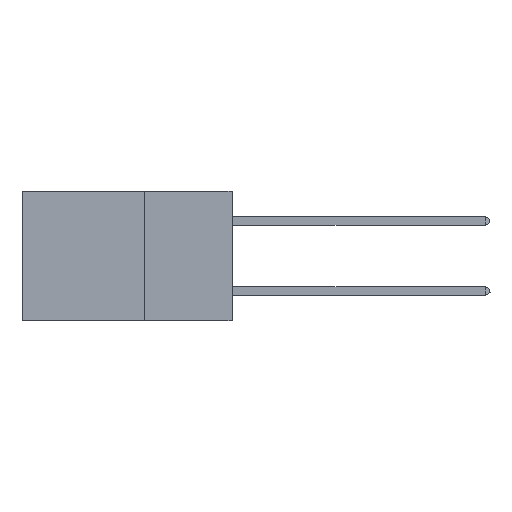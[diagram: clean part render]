
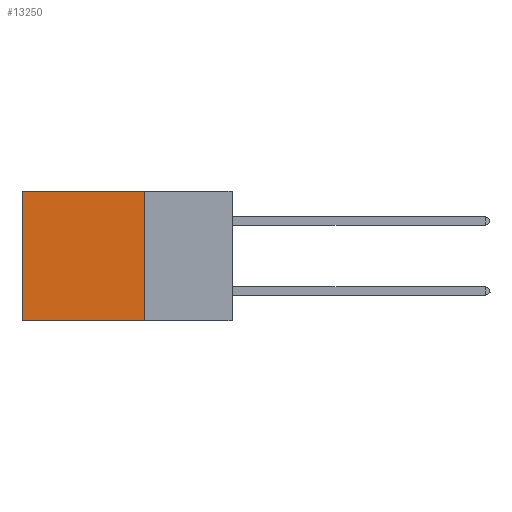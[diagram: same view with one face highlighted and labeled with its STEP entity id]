
A CAD part, left-side view. The second image highlights one B-rep face of the part: STEP entity #13250.
In plain terms, the highlighted planar face has unit normal (-1, 0, 0).
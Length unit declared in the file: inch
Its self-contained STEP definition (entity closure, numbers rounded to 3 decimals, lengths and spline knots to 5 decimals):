
#2627 = DIRECTION ( 'NONE',  ( 1., 0., 0. ) ) ;
#4089 = VECTOR ( 'NONE', #7491, 39.37008 ) ;
#6289 = CARTESIAN_POINT ( 'NONE',  ( 0.2875, 0.6, 0. ) ) ;
#6805 = EDGE_CURVE ( 'NONE', #7713, #23084, #10847, .T. ) ;
#7491 = DIRECTION ( 'NONE',  ( 0., 0., -1. ) ) ;
#7713 = VERTEX_POINT ( 'NONE', #10633 ) ;
#8462 = LINE ( 'NONE', #6289, #22477 ) ;
#8815 = CARTESIAN_POINT ( 'NONE',  ( 0.2875, 0.25, 0. ) ) ;
#8877 = ORIENTED_EDGE ( 'NONE', *, *, #18976, .T. ) ;
#9646 = VERTEX_POINT ( 'NONE', #8815 ) ;
#10633 = CARTESIAN_POINT ( 'NONE',  ( 0.2875, 0.25, -0.37 ) ) ;
#10847 = LINE ( 'NONE', #23865, #21742 ) ;
#12954 = EDGE_LOOP ( 'NONE', ( #18562, #14922, #18310, #8877 ) ) ;
#13250 = ADVANCED_FACE ( 'NONE', ( #20802 ), #13414, .F. ) ;
#13275 = DIRECTION ( 'NONE',  ( 0., 1., 0. ) ) ;
#13371 = LINE ( 'NONE', #17470, #16397 ) ;
#13414 = PLANE ( 'NONE',  #17568 ) ;
#14922 = ORIENTED_EDGE ( 'NONE', *, *, #6805, .F. ) ;
#15028 = DIRECTION ( 'NONE',  ( 0., 0., -1. ) ) ;
#15444 = VERTEX_POINT ( 'NONE', #25153 ) ;
#15495 = LINE ( 'NONE', #18174, #4089 ) ;
#16397 = VECTOR ( 'NONE', #13275, 39.37008 ) ;
#17170 = EDGE_CURVE ( 'NONE', #15444, #23084, #8462, .T. ) ;
#17470 = CARTESIAN_POINT ( 'NONE',  ( 0.2875, 0.25, 0. ) ) ;
#17510 = CARTESIAN_POINT ( 'NONE',  ( 0.2875, 0.25, 0. ) ) ;
#17527 = EDGE_CURVE ( 'NONE', #9646, #7713, #15495, .T. ) ;
#17568 = AXIS2_PLACEMENT_3D ( 'NONE', #17510, #2627, #17610 ) ;
#17610 = DIRECTION ( 'NONE',  ( 0., 0., -1. ) ) ;
#18174 = CARTESIAN_POINT ( 'NONE',  ( 0.2875, 0.25, 0. ) ) ;
#18310 = ORIENTED_EDGE ( 'NONE', *, *, #17527, .F. ) ;
#18562 = ORIENTED_EDGE ( 'NONE', *, *, #17170, .T. ) ;
#18976 = EDGE_CURVE ( 'NONE', #9646, #15444, #13371, .T. ) ;
#19697 = CARTESIAN_POINT ( 'NONE',  ( 0.2875, 0.6, -0.37 ) ) ;
#20802 = FACE_OUTER_BOUND ( 'NONE', #12954, .T. ) ;
#21742 = VECTOR ( 'NONE', #23769, 39.37008 ) ;
#22477 = VECTOR ( 'NONE', #15028, 39.37008 ) ;
#23084 = VERTEX_POINT ( 'NONE', #19697 ) ;
#23769 = DIRECTION ( 'NONE',  ( 0., 1., 0. ) ) ;
#23865 = CARTESIAN_POINT ( 'NONE',  ( 0.2875, 0.25, -0.37 ) ) ;
#25153 = CARTESIAN_POINT ( 'NONE',  ( 0.2875, 0.6, 0. ) ) ;
